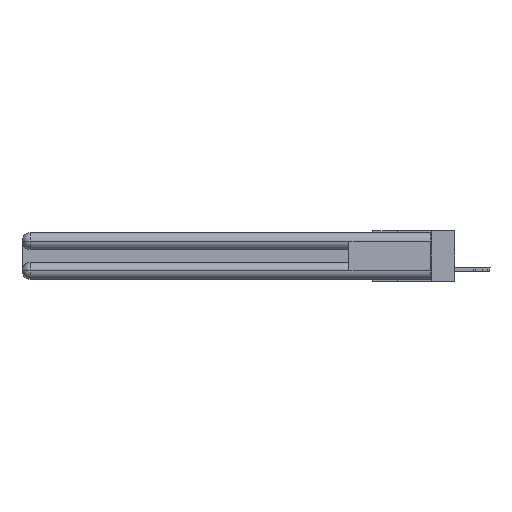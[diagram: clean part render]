
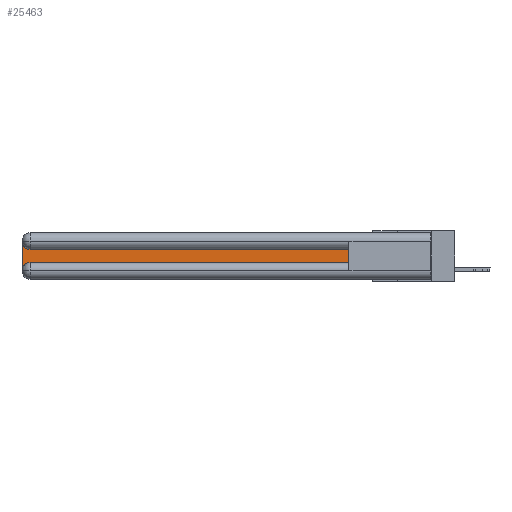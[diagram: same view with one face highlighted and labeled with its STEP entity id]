
A CAD part, left-side view. The second image highlights one B-rep face of the part: STEP entity #25463.
In plain terms, the highlighted planar face has unit normal (-1, 0, 0).
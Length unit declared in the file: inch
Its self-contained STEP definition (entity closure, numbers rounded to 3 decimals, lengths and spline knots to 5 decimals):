
#363 = VECTOR ( 'NONE', #2344, 39.37008 ) ;
#531 = EDGE_CURVE ( 'NONE', #27772, #14774, #26979, .T. ) ;
#908 = FACE_OUTER_BOUND ( 'NONE', #3717, .T. ) ;
#920 = DIRECTION ( 'NONE',  ( 0., -1., 0. ) ) ;
#1485 = ORIENTED_EDGE ( 'NONE', *, *, #9055, .T. ) ;
#2344 = DIRECTION ( 'NONE',  ( 0., 0., -1. ) ) ;
#2744 = CIRCLE ( 'NONE', #22711, 0.06 ) ;
#3688 = ORIENTED_EDGE ( 'NONE', *, *, #531, .T. ) ;
#3717 = EDGE_LOOP ( 'NONE', ( #12660, #13477, #28325, #6929, #3688, #1485 ) ) ;
#4501 = LINE ( 'NONE', #28182, #363 ) ;
#6029 = LINE ( 'NONE', #24451, #21837 ) ;
#6036 = AXIS2_PLACEMENT_3D ( 'NONE', #6426, #26173, #14745 ) ;
#6206 = VERTEX_POINT ( 'NONE', #16090 ) ;
#6426 = CARTESIAN_POINT ( 'NONE',  ( 0.075, 3., -0.1225 ) ) ;
#6929 = ORIENTED_EDGE ( 'NONE', *, *, #25415, .T. ) ;
#9055 = EDGE_CURVE ( 'NONE', #14774, #21610, #9980, .T. ) ;
#9980 = LINE ( 'NONE', #12578, #10676 ) ;
#10486 = DIRECTION ( 'NONE',  ( 0., 0., -1. ) ) ;
#10676 = VECTOR ( 'NONE', #28236, 39.37008 ) ;
#11551 = VERTEX_POINT ( 'NONE', #17051 ) ;
#11582 = DIRECTION ( 'NONE',  ( 1., 0., 0. ) ) ;
#12513 = EDGE_CURVE ( 'NONE', #21610, #13629, #6029, .T. ) ;
#12578 = CARTESIAN_POINT ( 'NONE',  ( 0.075, 0.6, -0.2175 ) ) ;
#12660 = ORIENTED_EDGE ( 'NONE', *, *, #12513, .T. ) ;
#13477 = ORIENTED_EDGE ( 'NONE', *, *, #22572, .T. ) ;
#13629 = VERTEX_POINT ( 'NONE', #15044 ) ;
#14745 = DIRECTION ( 'NONE',  ( 0., 0., -1. ) ) ;
#14774 = VERTEX_POINT ( 'NONE', #19702 ) ;
#14897 = CIRCLE ( 'NONE', #15391, 0.06 ) ;
#15011 = EDGE_CURVE ( 'NONE', #11551, #6206, #4501, .T. ) ;
#15044 = CARTESIAN_POINT ( 'NONE',  ( 0.075, 2.94, -0.1225 ) ) ;
#15282 = VECTOR ( 'NONE', #920, 39.37008 ) ;
#15391 = AXIS2_PLACEMENT_3D ( 'NONE', #21578, #19456, #10486 ) ;
#16090 = CARTESIAN_POINT ( 'NONE',  ( 0.075, 3., -0.2775 ) ) ;
#16179 = CARTESIAN_POINT ( 'NONE',  ( 0.075, 0.6, -0.1225 ) ) ;
#16307 = DIRECTION ( 'NONE',  ( 0., 0., -1. ) ) ;
#17051 = CARTESIAN_POINT ( 'NONE',  ( 0.075, 3., -0.0625 ) ) ;
#19456 = DIRECTION ( 'NONE',  ( 1., 0., 0. ) ) ;
#19702 = CARTESIAN_POINT ( 'NONE',  ( 0.075, 0.6, -0.2175 ) ) ;
#20376 = CARTESIAN_POINT ( 'NONE',  ( 0.075, 0.6, -0.2175 ) ) ;
#21578 = CARTESIAN_POINT ( 'NONE',  ( 0.075, 2.94, -0.2775 ) ) ;
#21610 = VERTEX_POINT ( 'NONE', #16179 ) ;
#21837 = VECTOR ( 'NONE', #24722, 39.37008 ) ;
#22221 = CARTESIAN_POINT ( 'NONE',  ( 0.075, 2.94, -0.2175 ) ) ;
#22572 = EDGE_CURVE ( 'NONE', #13629, #11551, #2744, .T. ) ;
#22711 = AXIS2_PLACEMENT_3D ( 'NONE', #27072, #11582, #16307 ) ;
#24451 = CARTESIAN_POINT ( 'NONE',  ( 0.075, 0.6, -0.1225 ) ) ;
#24722 = DIRECTION ( 'NONE',  ( 0., 1., 0. ) ) ;
#25415 = EDGE_CURVE ( 'NONE', #6206, #27772, #14897, .T. ) ;
#25463 = ADVANCED_FACE ( 'NONE', ( #908 ), #27973, .F. ) ;
#26173 = DIRECTION ( 'NONE',  ( 1., 0., 0. ) ) ;
#26979 = LINE ( 'NONE', #20376, #15282 ) ;
#27072 = CARTESIAN_POINT ( 'NONE',  ( 0.075, 2.94, -0.0625 ) ) ;
#27772 = VERTEX_POINT ( 'NONE', #22221 ) ;
#27973 = PLANE ( 'NONE',  #6036 ) ;
#28182 = CARTESIAN_POINT ( 'NONE',  ( 0.075, 3., -0.2175 ) ) ;
#28236 = DIRECTION ( 'NONE',  ( 0., 0., 1. ) ) ;
#28325 = ORIENTED_EDGE ( 'NONE', *, *, #15011, .T. ) ;
